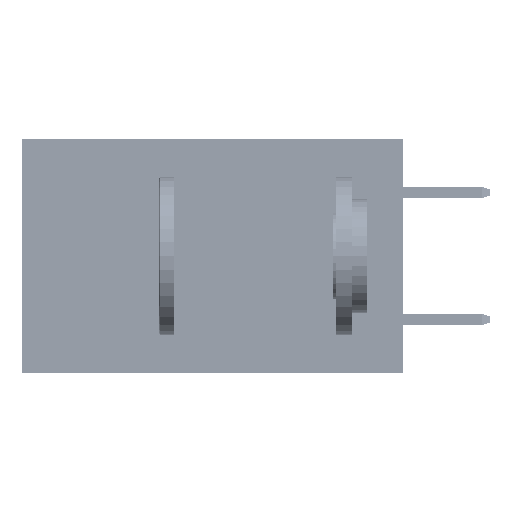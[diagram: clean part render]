
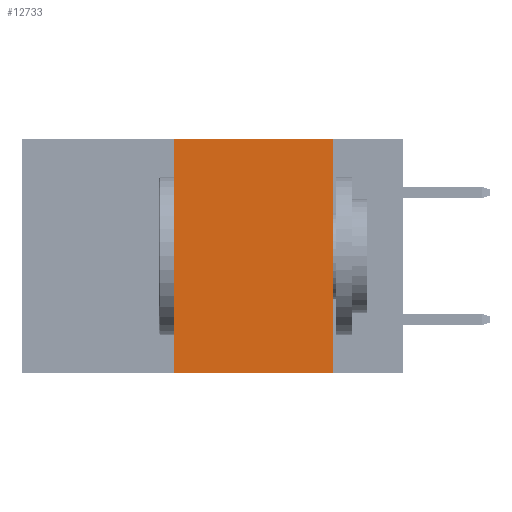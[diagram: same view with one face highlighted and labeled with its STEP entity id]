
A CAD part, left-side view. The second image highlights one B-rep face of the part: STEP entity #12733.
In plain terms, the highlighted planar face has unit normal (-1, 0, 0).
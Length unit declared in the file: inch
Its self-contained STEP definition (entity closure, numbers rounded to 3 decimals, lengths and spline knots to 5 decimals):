
#1662 = CARTESIAN_POINT ( 'NONE',  ( 0., 0.11, 0. ) ) ;
#2455 = PLANE ( 'NONE',  #47733 ) ;
#3983 = EDGE_CURVE ( 'NONE', #45287, #42731, #46425, .T. ) ;
#7013 = DIRECTION ( 'NONE',  ( 1., 0., 0. ) ) ;
#9290 = VECTOR ( 'NONE', #22445, 39.37008 ) ;
#10188 = LINE ( 'NONE', #39683, #24724 ) ;
#12733 = ADVANCED_FACE ( 'NONE', ( #35857 ), #2455, .F. ) ;
#12831 = VERTEX_POINT ( 'NONE', #30187 ) ;
#14255 = CARTESIAN_POINT ( 'NONE',  ( 0., 0.36, 0. ) ) ;
#15409 = VERTEX_POINT ( 'NONE', #25398 ) ;
#16210 = ORIENTED_EDGE ( 'NONE', *, *, #32601, .F. ) ;
#16228 = DIRECTION ( 'NONE',  ( 0., -1., 0. ) ) ;
#22445 = DIRECTION ( 'NONE',  ( 0., 0., 1. ) ) ;
#22939 = ORIENTED_EDGE ( 'NONE', *, *, #32703, .T. ) ;
#24601 = LINE ( 'NONE', #1662, #26251 ) ;
#24724 = VECTOR ( 'NONE', #47227, 39.37008 ) ;
#24920 = ORIENTED_EDGE ( 'NONE', *, *, #3983, .F. ) ;
#25398 = CARTESIAN_POINT ( 'NONE',  ( 0., 0.36, -0.37 ) ) ;
#25566 = CARTESIAN_POINT ( 'NONE',  ( 0., 0.6, 0. ) ) ;
#26105 = LINE ( 'NONE', #30245, #9290 ) ;
#26251 = VECTOR ( 'NONE', #31645, 39.37008 ) ;
#27672 = CARTESIAN_POINT ( 'NONE',  ( 0., 0.6, 0. ) ) ;
#30187 = CARTESIAN_POINT ( 'NONE',  ( 0., 0.11, -0.37 ) ) ;
#30245 = CARTESIAN_POINT ( 'NONE',  ( 0., 0.36, 0. ) ) ;
#31645 = DIRECTION ( 'NONE',  ( 0., 0., -1. ) ) ;
#32601 = EDGE_CURVE ( 'NONE', #42731, #12831, #24601, .T. ) ;
#32703 = EDGE_CURVE ( 'NONE', #15409, #12831, #10188, .T. ) ;
#33095 = DIRECTION ( 'NONE',  ( 0., 0., -1. ) ) ;
#33430 = ORIENTED_EDGE ( 'NONE', *, *, #35574, .F. ) ;
#35574 = EDGE_CURVE ( 'NONE', #15409, #45287, #26105, .T. ) ;
#35857 = FACE_OUTER_BOUND ( 'NONE', #43356, .T. ) ;
#39683 = CARTESIAN_POINT ( 'NONE',  ( 0., 0.6, -0.37 ) ) ;
#40263 = VECTOR ( 'NONE', #16228, 39.37008 ) ;
#41499 = CARTESIAN_POINT ( 'NONE',  ( 0., 0.11, 0. ) ) ;
#42731 = VERTEX_POINT ( 'NONE', #41499 ) ;
#43356 = EDGE_LOOP ( 'NONE', ( #16210, #24920, #33430, #22939 ) ) ;
#45287 = VERTEX_POINT ( 'NONE', #14255 ) ;
#46425 = LINE ( 'NONE', #27672, #40263 ) ;
#47227 = DIRECTION ( 'NONE',  ( 0., -1., 0. ) ) ;
#47733 = AXIS2_PLACEMENT_3D ( 'NONE', #25566, #7013, #33095 ) ;
